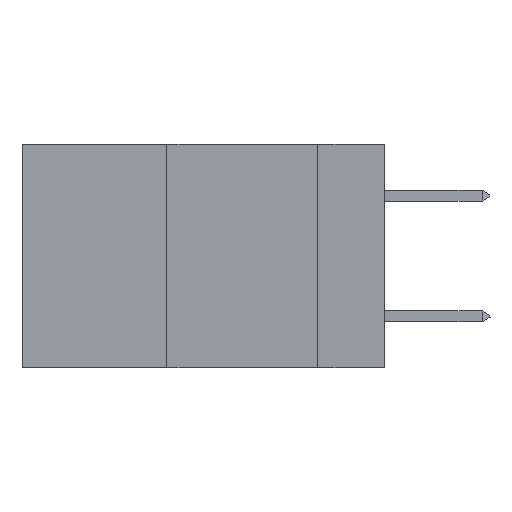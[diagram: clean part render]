
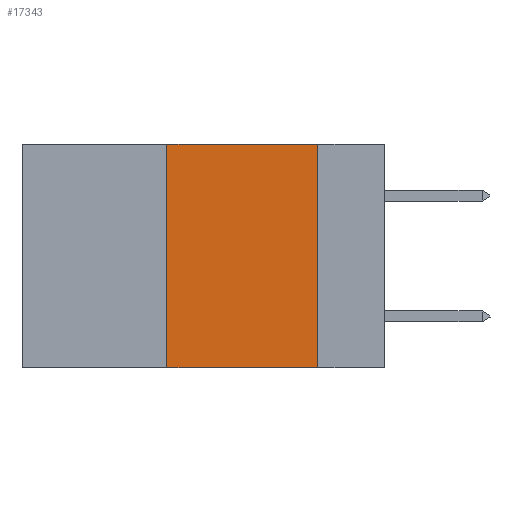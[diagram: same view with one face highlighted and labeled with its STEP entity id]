
A CAD part, left-side view. The second image highlights one B-rep face of the part: STEP entity #17343.
In plain terms, the highlighted planar face has unit normal (-1, 0, 0).
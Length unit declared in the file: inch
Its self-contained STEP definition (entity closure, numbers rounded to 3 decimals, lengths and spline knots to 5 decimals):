
#178 = CARTESIAN_POINT ( 'NONE',  ( 0., 0.11, -0.37 ) ) ;
#2045 = EDGE_LOOP ( 'NONE', ( #22538, #8407, #16573, #27969 ) ) ;
#3851 = CARTESIAN_POINT ( 'NONE',  ( 0., 0.6, 0. ) ) ;
#4400 = EDGE_CURVE ( 'NONE', #6706, #5319, #9110, .T. ) ;
#4511 = VERTEX_POINT ( 'NONE', #178 ) ;
#5319 = VERTEX_POINT ( 'NONE', #5965 ) ;
#5965 = CARTESIAN_POINT ( 'NONE',  ( 0., 0.11, 0. ) ) ;
#6706 = VERTEX_POINT ( 'NONE', #26299 ) ;
#8407 = ORIENTED_EDGE ( 'NONE', *, *, #4400, .F. ) ;
#9110 = LINE ( 'NONE', #3851, #14043 ) ;
#9945 = DIRECTION ( 'NONE',  ( 0., -1., 0. ) ) ;
#10367 = VECTOR ( 'NONE', #40334, 39.37008 ) ;
#10445 = DIRECTION ( 'NONE',  ( 0., 0., 1. ) ) ;
#11015 = CARTESIAN_POINT ( 'NONE',  ( 0., 0.36, -0.37 ) ) ;
#11410 = EDGE_CURVE ( 'NONE', #16835, #6706, #37583, .T. ) ;
#11830 = LINE ( 'NONE', #27253, #10367 ) ;
#12740 = FACE_OUTER_BOUND ( 'NONE', #2045, .T. ) ;
#13138 = CARTESIAN_POINT ( 'NONE',  ( 0., 0.6, 0. ) ) ;
#13770 = AXIS2_PLACEMENT_3D ( 'NONE', #13138, #22881, #35428 ) ;
#14043 = VECTOR ( 'NONE', #9945, 39.37008 ) ;
#14784 = EDGE_CURVE ( 'NONE', #5319, #4511, #27572, .T. ) ;
#15335 = VECTOR ( 'NONE', #37537, 39.37008 ) ;
#16573 = ORIENTED_EDGE ( 'NONE', *, *, #11410, .F. ) ;
#16835 = VERTEX_POINT ( 'NONE', #11015 ) ;
#17343 = ADVANCED_FACE ( 'NONE', ( #12740 ), #19737, .F. ) ;
#19737 = PLANE ( 'NONE',  #13770 ) ;
#22538 = ORIENTED_EDGE ( 'NONE', *, *, #14784, .F. ) ;
#22881 = DIRECTION ( 'NONE',  ( 1., 0., 0. ) ) ;
#24848 = CARTESIAN_POINT ( 'NONE',  ( 0., 0.11, 0. ) ) ;
#26299 = CARTESIAN_POINT ( 'NONE',  ( 0., 0.36, 0. ) ) ;
#26873 = VECTOR ( 'NONE', #10445, 39.37008 ) ;
#27253 = CARTESIAN_POINT ( 'NONE',  ( 0., 0.6, -0.37 ) ) ;
#27572 = LINE ( 'NONE', #24848, #15335 ) ;
#27969 = ORIENTED_EDGE ( 'NONE', *, *, #34483, .T. ) ;
#29193 = CARTESIAN_POINT ( 'NONE',  ( 0., 0.36, 0. ) ) ;
#34483 = EDGE_CURVE ( 'NONE', #16835, #4511, #11830, .T. ) ;
#35428 = DIRECTION ( 'NONE',  ( 0., 0., -1. ) ) ;
#37537 = DIRECTION ( 'NONE',  ( 0., 0., -1. ) ) ;
#37583 = LINE ( 'NONE', #29193, #26873 ) ;
#40334 = DIRECTION ( 'NONE',  ( 0., -1., 0. ) ) ;
